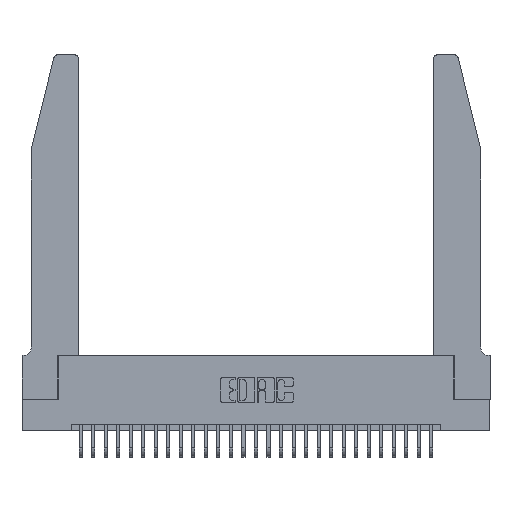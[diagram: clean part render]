
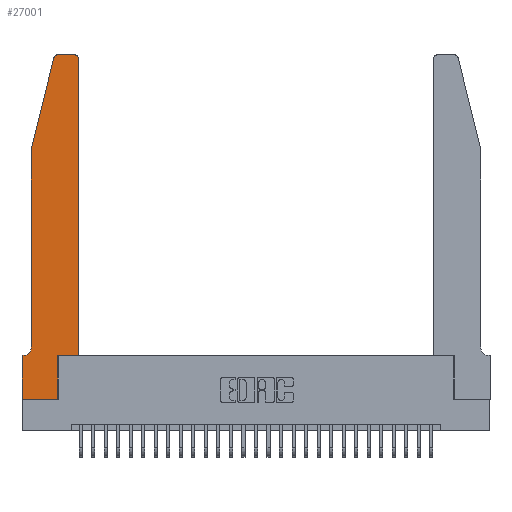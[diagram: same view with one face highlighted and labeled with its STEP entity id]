
A CAD part, top view. The second image highlights one B-rep face of the part: STEP entity #27001.
In plain terms, the highlighted planar face has unit normal (0, 0, 1).
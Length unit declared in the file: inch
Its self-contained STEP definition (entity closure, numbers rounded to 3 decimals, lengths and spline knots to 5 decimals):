
#208 = EDGE_CURVE ( 'NONE', #29019, #19413, #18742, .T. ) ;
#247 = CARTESIAN_POINT ( 'NONE',  ( 0.4505, 0.35, 0.37 ) ) ;
#418 = ORIENTED_EDGE ( 'NONE', *, *, #25882, .T. ) ;
#530 = EDGE_CURVE ( 'NONE', #23054, #22034, #23204, .T. ) ;
#778 = CARTESIAN_POINT ( 'NONE',  ( 0.0755, 2., 0.37 ) ) ;
#1096 = VECTOR ( 'NONE', #24043, 39.37008 ) ;
#1300 = AXIS2_PLACEMENT_3D ( 'NONE', #19983, #10418, #25341 ) ;
#2147 = EDGE_LOOP ( 'NONE', ( #8764, #2249, #19709, #14799, #8606, #10474, #6885, #418, #19753, #10845, #2664, #2841 ) ) ;
#2249 = ORIENTED_EDGE ( 'NONE', *, *, #530, .T. ) ;
#2664 = ORIENTED_EDGE ( 'NONE', *, *, #5873, .T. ) ;
#2841 = ORIENTED_EDGE ( 'NONE', *, *, #30829, .T. ) ;
#3796 = DIRECTION ( 'NONE',  ( 0., 0., -1. ) ) ;
#4079 = DIRECTION ( 'NONE',  ( 1., 0., 0. ) ) ;
#4102 = CIRCLE ( 'NONE', #13938, 0.07 ) ;
#4211 = CARTESIAN_POINT ( 'NONE',  ( 0., 0., 0.37 ) ) ;
#4888 = CARTESIAN_POINT ( 'NONE',  ( 0.0755, 0.35, 0.37 ) ) ;
#5873 = EDGE_CURVE ( 'NONE', #23163, #10966, #9653, .T. ) ;
#6178 = DIRECTION ( 'NONE',  ( 0., 0., 1. ) ) ;
#6362 = DIRECTION ( 'NONE',  ( 0., 1., 0. ) ) ;
#6885 = ORIENTED_EDGE ( 'NONE', *, *, #17620, .T. ) ;
#7402 = CARTESIAN_POINT ( 'NONE',  ( 0.25487, 2.72718, 0.37 ) ) ;
#7615 = VECTOR ( 'NONE', #17170, 39.37008 ) ;
#7919 = CARTESIAN_POINT ( 'NONE',  ( 0.0755, 0.42, 0.37 ) ) ;
#8075 = VERTEX_POINT ( 'NONE', #8680 ) ;
#8520 = LINE ( 'NONE', #21613, #1096 ) ;
#8606 = ORIENTED_EDGE ( 'NONE', *, *, #11084, .T. ) ;
#8680 = CARTESIAN_POINT ( 'NONE',  ( 0.2865, 0.35, 0.37 ) ) ;
#8764 = ORIENTED_EDGE ( 'NONE', *, *, #19691, .T. ) ;
#9570 = DIRECTION ( 'NONE',  ( -1., 0., 0. ) ) ;
#9625 = DIRECTION ( 'NONE',  ( 1., 0., 0. ) ) ;
#9653 = LINE ( 'NONE', #30151, #28703 ) ;
#10418 = DIRECTION ( 'NONE',  ( 0., 0., 1. ) ) ;
#10474 = ORIENTED_EDGE ( 'NONE', *, *, #208, .T. ) ;
#10845 = ORIENTED_EDGE ( 'NONE', *, *, #20431, .T. ) ;
#10966 = VERTEX_POINT ( 'NONE', #12829 ) ;
#11084 = EDGE_CURVE ( 'NONE', #13981, #29019, #4102, .T. ) ;
#11396 = CARTESIAN_POINT ( 'NONE',  ( 0.0055, 0.35, 0.37 ) ) ;
#11795 = DIRECTION ( 'NONE',  ( -1., 0., 0. ) ) ;
#11946 = VERTEX_POINT ( 'NONE', #23414 ) ;
#12024 = AXIS2_PLACEMENT_3D ( 'NONE', #27808, #13528, #16005 ) ;
#12788 = CIRCLE ( 'NONE', #14634, 0.03 ) ;
#12829 = CARTESIAN_POINT ( 'NONE',  ( 0.4505, 2.72, 0.37 ) ) ;
#13364 = CARTESIAN_POINT ( 'NONE',  ( 0.4205, 2.72, 0.37 ) ) ;
#13528 = DIRECTION ( 'NONE',  ( 0., 0., 1. ) ) ;
#13779 = CARTESIAN_POINT ( 'NONE',  ( 0., 0., 0.37 ) ) ;
#13938 = AXIS2_PLACEMENT_3D ( 'NONE', #18386, #3796, #9570 ) ;
#13981 = VERTEX_POINT ( 'NONE', #7919 ) ;
#14529 = LINE ( 'NONE', #15833, #16008 ) ;
#14634 = AXIS2_PLACEMENT_3D ( 'NONE', #13364, #6178, #4079 ) ;
#14799 = ORIENTED_EDGE ( 'NONE', *, *, #26257, .T. ) ;
#14939 = VECTOR ( 'NONE', #23463, 39.37008 ) ;
#15384 = VECTOR ( 'NONE', #11795, 39.37008 ) ;
#15513 = DIRECTION ( 'NONE',  ( 0., -1., 0. ) ) ;
#15694 = PLANE ( 'NONE',  #12024 ) ;
#15734 = DIRECTION ( 'NONE',  ( -1., 0., 0. ) ) ;
#15833 = CARTESIAN_POINT ( 'NONE',  ( 0.0755, 2., 0.37 ) ) ;
#16005 = DIRECTION ( 'NONE',  ( 1., 0., 0. ) ) ;
#16008 = VECTOR ( 'NONE', #15513, 39.37008 ) ;
#16349 = CARTESIAN_POINT ( 'NONE',  ( 0., 0.35, 0.37 ) ) ;
#17170 = DIRECTION ( 'NONE',  ( 0., 1., 0. ) ) ;
#17620 = EDGE_CURVE ( 'NONE', #19413, #22697, #23546, .T. ) ;
#18386 = CARTESIAN_POINT ( 'NONE',  ( 0.0055, 0.42, 0.37 ) ) ;
#18742 = LINE ( 'NONE', #4888, #15384 ) ;
#18840 = VERTEX_POINT ( 'NONE', #21444 ) ;
#19413 = VERTEX_POINT ( 'NONE', #16349 ) ;
#19494 = LINE ( 'NONE', #778, #22461 ) ;
#19691 = EDGE_CURVE ( 'NONE', #11946, #23054, #29557, .T. ) ;
#19709 = ORIENTED_EDGE ( 'NONE', *, *, #30557, .T. ) ;
#19753 = ORIENTED_EDGE ( 'NONE', *, *, #30353, .T. ) ;
#19983 = CARTESIAN_POINT ( 'NONE',  ( 0.284, 2.72, 0.37 ) ) ;
#20115 = FACE_OUTER_BOUND ( 'NONE', #2147, .T. ) ;
#20431 = EDGE_CURVE ( 'NONE', #8075, #23163, #8520, .T. ) ;
#21444 = CARTESIAN_POINT ( 'NONE',  ( 0.2865, 0., 0.37 ) ) ;
#21524 = CARTESIAN_POINT ( 'NONE',  ( 0.0755, 2., 0.37 ) ) ;
#21613 = CARTESIAN_POINT ( 'NONE',  ( 0.4505, 0.35, 0.37 ) ) ;
#22034 = VERTEX_POINT ( 'NONE', #7402 ) ;
#22189 = VERTEX_POINT ( 'NONE', #21524 ) ;
#22461 = VECTOR ( 'NONE', #24449, 39.37008 ) ;
#22697 = VERTEX_POINT ( 'NONE', #13779 ) ;
#23054 = VERTEX_POINT ( 'NONE', #30853 ) ;
#23150 = VECTOR ( 'NONE', #15734, 39.37008 ) ;
#23163 = VERTEX_POINT ( 'NONE', #247 ) ;
#23204 = CIRCLE ( 'NONE', #1300, 0.03 ) ;
#23414 = CARTESIAN_POINT ( 'NONE',  ( 0.4205, 2.75, 0.37 ) ) ;
#23463 = DIRECTION ( 'NONE',  ( 0., -1., 0. ) ) ;
#23546 = LINE ( 'NONE', #25675, #14939 ) ;
#24043 = DIRECTION ( 'NONE',  ( 1., 0., 0. ) ) ;
#24449 = DIRECTION ( 'NONE',  ( -0.239, -0.971, 0. ) ) ;
#24710 = CARTESIAN_POINT ( 'NONE',  ( 0.2865, 0.35, 0.37 ) ) ;
#25152 = LINE ( 'NONE', #24710, #7615 ) ;
#25341 = DIRECTION ( 'NONE',  ( 1., 0., 0. ) ) ;
#25368 = CARTESIAN_POINT ( 'NONE',  ( 0.2605, 2.75, 0.37 ) ) ;
#25675 = CARTESIAN_POINT ( 'NONE',  ( 0., 0., 0.37 ) ) ;
#25882 = EDGE_CURVE ( 'NONE', #22697, #18840, #28385, .T. ) ;
#26257 = EDGE_CURVE ( 'NONE', #22189, #13981, #14529, .T. ) ;
#27001 = ADVANCED_FACE ( 'NONE', ( #20115 ), #15694, .T. ) ;
#27808 = CARTESIAN_POINT ( 'NONE',  ( 0., 0.35, 0.37 ) ) ;
#28385 = LINE ( 'NONE', #4211, #29884 ) ;
#28703 = VECTOR ( 'NONE', #6362, 39.37008 ) ;
#29019 = VERTEX_POINT ( 'NONE', #11396 ) ;
#29557 = LINE ( 'NONE', #25368, #23150 ) ;
#29884 = VECTOR ( 'NONE', #9625, 39.37008 ) ;
#30151 = CARTESIAN_POINT ( 'NONE',  ( 0.4505, 0.35, 0.37 ) ) ;
#30353 = EDGE_CURVE ( 'NONE', #18840, #8075, #25152, .T. ) ;
#30557 = EDGE_CURVE ( 'NONE', #22034, #22189, #19494, .T. ) ;
#30829 = EDGE_CURVE ( 'NONE', #10966, #11946, #12788, .T. ) ;
#30853 = CARTESIAN_POINT ( 'NONE',  ( 0.284, 2.75, 0.37 ) ) ;
